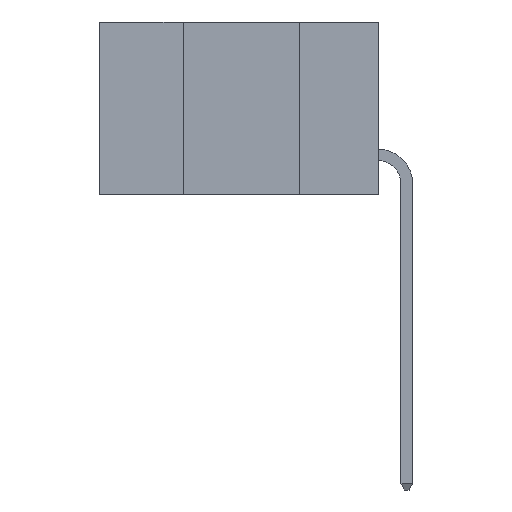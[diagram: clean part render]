
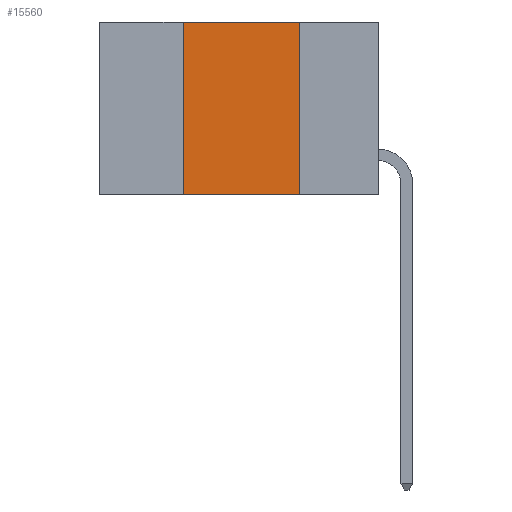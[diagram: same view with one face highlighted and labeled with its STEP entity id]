
A CAD part, left-side view. The second image highlights one B-rep face of the part: STEP entity #15560.
In plain terms, the highlighted planar face has unit normal (-1, 0, 0).
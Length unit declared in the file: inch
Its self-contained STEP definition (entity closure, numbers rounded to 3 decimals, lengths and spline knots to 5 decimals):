
#600 = ORIENTED_EDGE ( 'NONE', *, *, #8456, .T. ) ;
#1450 = EDGE_CURVE ( 'NONE', #3718, #12063, #13771, .T. ) ;
#1670 = CARTESIAN_POINT ( 'NONE',  ( 0., 0.42, 0. ) ) ;
#3449 = CARTESIAN_POINT ( 'NONE',  ( 0., 0.6, 0. ) ) ;
#3718 = VERTEX_POINT ( 'NONE', #11301 ) ;
#4056 = LINE ( 'NONE', #5894, #12907 ) ;
#4221 = CARTESIAN_POINT ( 'NONE',  ( 0., 0.42, -0.37 ) ) ;
#4509 = VERTEX_POINT ( 'NONE', #1670 ) ;
#4731 = DIRECTION ( 'NONE',  ( 0., 0., -1. ) ) ;
#5271 = LINE ( 'NONE', #13725, #11303 ) ;
#5894 = CARTESIAN_POINT ( 'NONE',  ( 0., 0.6, -0.37 ) ) ;
#5947 = DIRECTION ( 'NONE',  ( 0., -1., 0. ) ) ;
#7086 = CARTESIAN_POINT ( 'NONE',  ( 0., 0.6, 0. ) ) ;
#7479 = VECTOR ( 'NONE', #8193, 39.37008 ) ;
#7573 = EDGE_CURVE ( 'NONE', #11879, #4509, #5271, .T. ) ;
#7598 = EDGE_LOOP ( 'NONE', ( #12571, #12031, #11664, #600 ) ) ;
#7843 = DIRECTION ( 'NONE',  ( 0., 0., 1. ) ) ;
#8193 = DIRECTION ( 'NONE',  ( 0., 0., -1. ) ) ;
#8456 = EDGE_CURVE ( 'NONE', #11879, #12063, #4056, .T. ) ;
#9581 = PLANE ( 'NONE',  #10146 ) ;
#10146 = AXIS2_PLACEMENT_3D ( 'NONE', #3449, #11954, #4731 ) ;
#11301 = CARTESIAN_POINT ( 'NONE',  ( 0., 0.17, 0. ) ) ;
#11303 = VECTOR ( 'NONE', #7843, 39.37008 ) ;
#11664 = ORIENTED_EDGE ( 'NONE', *, *, #7573, .F. ) ;
#11809 = LINE ( 'NONE', #7086, #13815 ) ;
#11879 = VERTEX_POINT ( 'NONE', #4221 ) ;
#11954 = DIRECTION ( 'NONE',  ( 1., 0., 0. ) ) ;
#12031 = ORIENTED_EDGE ( 'NONE', *, *, #14745, .F. ) ;
#12063 = VERTEX_POINT ( 'NONE', #12947 ) ;
#12571 = ORIENTED_EDGE ( 'NONE', *, *, #1450, .F. ) ;
#12907 = VECTOR ( 'NONE', #15310, 39.37008 ) ;
#12947 = CARTESIAN_POINT ( 'NONE',  ( 0., 0.17, -0.37 ) ) ;
#13725 = CARTESIAN_POINT ( 'NONE',  ( 0., 0.42, -0.37 ) ) ;
#13771 = LINE ( 'NONE', #15322, #7479 ) ;
#13815 = VECTOR ( 'NONE', #5947, 39.37008 ) ;
#14317 = FACE_OUTER_BOUND ( 'NONE', #7598, .T. ) ;
#14745 = EDGE_CURVE ( 'NONE', #4509, #3718, #11809, .T. ) ;
#15310 = DIRECTION ( 'NONE',  ( 0., -1., 0. ) ) ;
#15322 = CARTESIAN_POINT ( 'NONE',  ( 0., 0.17, -0.37 ) ) ;
#15560 = ADVANCED_FACE ( 'NONE', ( #14317 ), #9581, .F. ) ;
